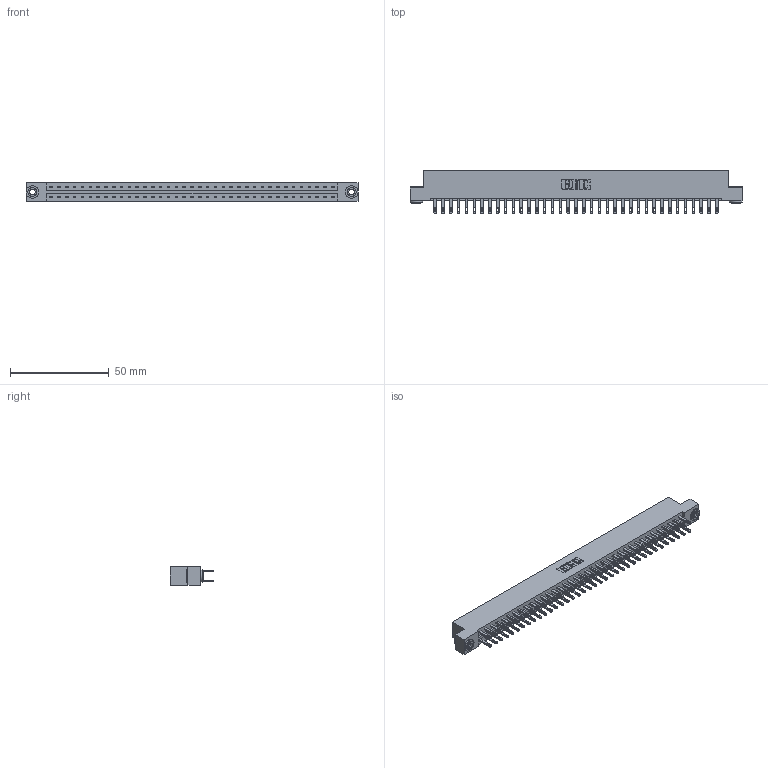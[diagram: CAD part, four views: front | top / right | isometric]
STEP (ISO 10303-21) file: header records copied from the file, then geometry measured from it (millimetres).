
FILE_DESCRIPTION (( 'STEP AP203' ), '1' );
FILE_NAME ('833-074-500-203.STEP', '2020-06-05T15:22:53', ( '' ), ( '' ), 'SwSTEP 2.0', 'SolidWorks 2020', '' );
FILE_SCHEMA (( 'CONFIG_CONTROL_DESIGN' ));
Length unit declared in the file: inch
Products named in the file (4): 833 Part_Flush - .156 Dia - TH; 345-292-001_345-293-100; 833-074-500-203; 345-250-002_345-250-002-102
Assembly tree (77 placements, depth 2):
  833-074-500-203
    833 Part_Flush - .156 Dia - TH
    345-292-001_345-293-100  x74
    345-250-002_345-250-002-102  x2
Bounding box: 168.15 x 21.85 x 9.4 mm (x, y, z)
Volume: 17365.7 mm3; surface area: 21512.1 mm2
Topology: 77 solids, 77 shells, 3704 faces, 11265 edges, 7506 vertices
Faces by surface type: plane 2300, cylinder 1396, cone 8
Entity records: 25030 total; most frequent: CARTESIAN_POINT 4129, ORIENTED_EDGE 4058, DIRECTION 3571, EDGE_CURVE 2029, LINE 1873, VECTOR 1873, VERTEX_POINT 1350, AXIS2_PLACEMENT_3D 849
